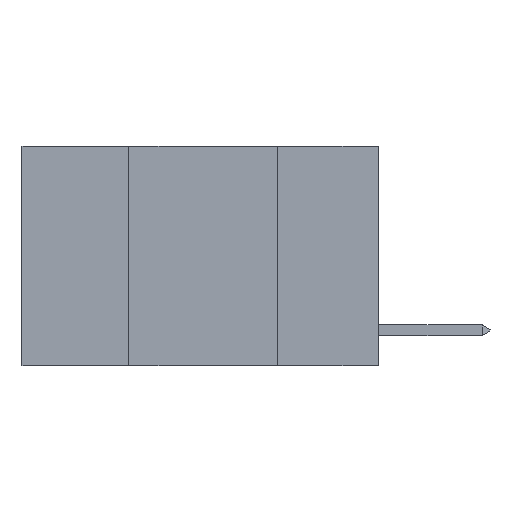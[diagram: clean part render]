
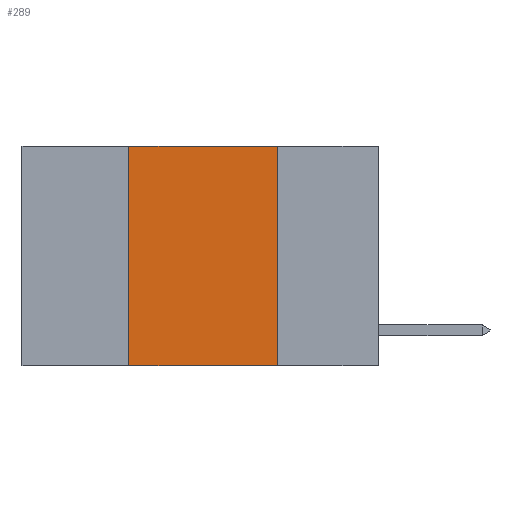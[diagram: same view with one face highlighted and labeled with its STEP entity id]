
A CAD part, left-side view. The second image highlights one B-rep face of the part: STEP entity #289.
In plain terms, the highlighted planar face has unit normal (-1, 0, 0).
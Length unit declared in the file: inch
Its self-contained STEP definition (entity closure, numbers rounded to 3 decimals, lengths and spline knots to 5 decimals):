
#289 = ADVANCED_FACE ( 'NONE', ( #4536 ), #7364, .F. ) ;
#564 = LINE ( 'NONE', #9027, #4594 ) ;
#570 = DIRECTION ( 'NONE',  ( 0., 0., -1. ) ) ;
#835 = LINE ( 'NONE', #3622, #9035 ) ;
#1943 = CARTESIAN_POINT ( 'NONE',  ( 0., 0.17, -0.37 ) ) ;
#2149 = ORIENTED_EDGE ( 'NONE', *, *, #7072, .T. ) ;
#3028 = VERTEX_POINT ( 'NONE', #8979 ) ;
#3070 = CARTESIAN_POINT ( 'NONE',  ( 0., 0.6, 0. ) ) ;
#3484 = EDGE_LOOP ( 'NONE', ( #7712, #7146, #10141, #2149 ) ) ;
#3622 = CARTESIAN_POINT ( 'NONE',  ( 0., 0.17, 0. ) ) ;
#3772 = CARTESIAN_POINT ( 'NONE',  ( 0., 0.17, 0. ) ) ;
#4536 = FACE_OUTER_BOUND ( 'NONE', #3484, .T. ) ;
#4594 = VECTOR ( 'NONE', #8985, 39.37008 ) ;
#4655 = VERTEX_POINT ( 'NONE', #1943 ) ;
#4828 = CARTESIAN_POINT ( 'NONE',  ( 0., 0.6, -0.37 ) ) ;
#4988 = VERTEX_POINT ( 'NONE', #3772 ) ;
#4995 = LINE ( 'NONE', #4828, #5597 ) ;
#5597 = VECTOR ( 'NONE', #8666, 39.37008 ) ;
#6143 = EDGE_CURVE ( 'NONE', #6439, #4988, #6796, .T. ) ;
#6179 = EDGE_CURVE ( 'NONE', #3028, #6439, #564, .T. ) ;
#6186 = VECTOR ( 'NONE', #7845, 39.37008 ) ;
#6439 = VERTEX_POINT ( 'NONE', #8645 ) ;
#6562 = DIRECTION ( 'NONE',  ( 0., 0., -1. ) ) ;
#6796 = LINE ( 'NONE', #3070, #6186 ) ;
#7072 = EDGE_CURVE ( 'NONE', #3028, #4655, #4995, .T. ) ;
#7146 = ORIENTED_EDGE ( 'NONE', *, *, #6143, .F. ) ;
#7239 = AXIS2_PLACEMENT_3D ( 'NONE', #9736, #8854, #6562 ) ;
#7364 = PLANE ( 'NONE',  #7239 ) ;
#7712 = ORIENTED_EDGE ( 'NONE', *, *, #8662, .F. ) ;
#7845 = DIRECTION ( 'NONE',  ( 0., -1., 0. ) ) ;
#8645 = CARTESIAN_POINT ( 'NONE',  ( 0., 0.42, 0. ) ) ;
#8662 = EDGE_CURVE ( 'NONE', #4988, #4655, #835, .T. ) ;
#8666 = DIRECTION ( 'NONE',  ( 0., -1., 0. ) ) ;
#8854 = DIRECTION ( 'NONE',  ( 1., 0., 0. ) ) ;
#8979 = CARTESIAN_POINT ( 'NONE',  ( 0., 0.42, -0.37 ) ) ;
#8985 = DIRECTION ( 'NONE',  ( 0., 0., 1. ) ) ;
#9027 = CARTESIAN_POINT ( 'NONE',  ( 0., 0.42, 0. ) ) ;
#9035 = VECTOR ( 'NONE', #570, 39.37008 ) ;
#9736 = CARTESIAN_POINT ( 'NONE',  ( 0., 0.6, 0. ) ) ;
#10141 = ORIENTED_EDGE ( 'NONE', *, *, #6179, .F. ) ;
